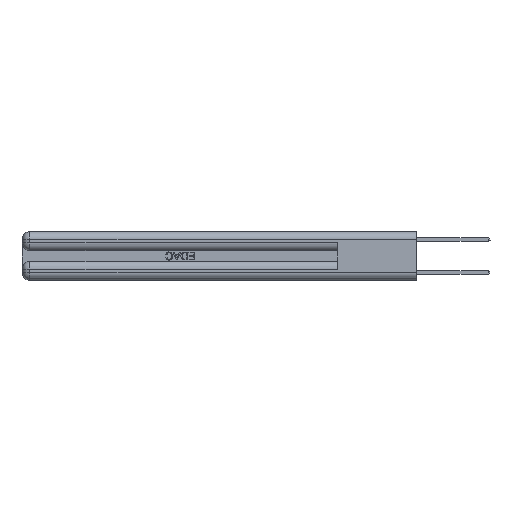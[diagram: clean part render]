
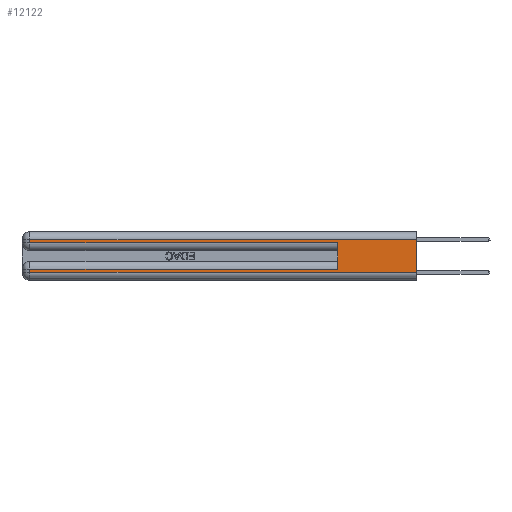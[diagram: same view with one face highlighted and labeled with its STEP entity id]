
A CAD part, left-side view. The second image highlights one B-rep face of the part: STEP entity #12122.
In plain terms, the highlighted planar face has unit normal (-1, 0, 0).
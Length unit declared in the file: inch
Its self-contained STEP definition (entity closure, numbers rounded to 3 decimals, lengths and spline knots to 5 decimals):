
#159 = CARTESIAN_POINT ( 'NONE',  ( 0., 2.94, 0.37 ) ) ;
#1840 = DIRECTION ( 'NONE',  ( 0., -1., 0. ) ) ;
#2116 = DIRECTION ( 'NONE',  ( 0., 1., 0. ) ) ;
#2978 = CARTESIAN_POINT ( 'NONE',  ( 0., 0., 0.285 ) ) ;
#3517 = VECTOR ( 'NONE', #26111, 39.37008 ) ;
#3708 = ORIENTED_EDGE ( 'NONE', *, *, #5303, .T. ) ;
#3730 = EDGE_CURVE ( 'NONE', #18620, #20975, #27559, .T. ) ;
#4450 = ORIENTED_EDGE ( 'NONE', *, *, #28834, .T. ) ;
#4956 = ORIENTED_EDGE ( 'NONE', *, *, #3730, .F. ) ;
#5303 = EDGE_CURVE ( 'NONE', #19756, #13577, #11422, .T. ) ;
#5795 = CARTESIAN_POINT ( 'NONE',  ( 0., 2.94, 0.31 ) ) ;
#6898 = VECTOR ( 'NONE', #15519, 39.37008 ) ;
#7164 = EDGE_CURVE ( 'NONE', #19826, #19756, #14748, .T. ) ;
#7222 = DIRECTION ( 'NONE',  ( 1., 0., 0. ) ) ;
#7768 = CARTESIAN_POINT ( 'NONE',  ( 0., 0.6, 0.285 ) ) ;
#8004 = LINE ( 'NONE', #22572, #20672 ) ;
#11073 = VECTOR ( 'NONE', #16482, 39.37008 ) ;
#11174 = EDGE_CURVE ( 'NONE', #24193, #13577, #8004, .T. ) ;
#11422 = LINE ( 'NONE', #15305, #14850 ) ;
#12122 = ADVANCED_FACE ( 'NONE', ( #18908 ), #23334, .F. ) ;
#12158 = DIRECTION ( 'NONE',  ( 0., 0., -1. ) ) ;
#13145 = ORIENTED_EDGE ( 'NONE', *, *, #7164, .T. ) ;
#13299 = EDGE_CURVE ( 'NONE', #18620, #19826, #31408, .T. ) ;
#13577 = VERTEX_POINT ( 'NONE', #32786 ) ;
#14748 = LINE ( 'NONE', #30093, #24421 ) ;
#14850 = VECTOR ( 'NONE', #1840, 39.37008 ) ;
#15305 = CARTESIAN_POINT ( 'NONE',  ( 0., 0., 0.06 ) ) ;
#15519 = DIRECTION ( 'NONE',  ( 0., 1., 0. ) ) ;
#16013 = VERTEX_POINT ( 'NONE', #28511 ) ;
#16149 = DIRECTION ( 'NONE',  ( 0., 0., 1. ) ) ;
#16348 = VECTOR ( 'NONE', #2116, 39.37008 ) ;
#16482 = DIRECTION ( 'NONE',  ( 0., -1., 0. ) ) ;
#18620 = VERTEX_POINT ( 'NONE', #21579 ) ;
#18908 = FACE_OUTER_BOUND ( 'NONE', #25288, .T. ) ;
#18922 = CARTESIAN_POINT ( 'NONE',  ( 0., 0.6, 0.145 ) ) ;
#19756 = VERTEX_POINT ( 'NONE', #27786 ) ;
#19826 = VERTEX_POINT ( 'NONE', #28006 ) ;
#20258 = DIRECTION ( 'NONE',  ( 0., 0., -1. ) ) ;
#20407 = CARTESIAN_POINT ( 'NONE',  ( 0., 0., 0.085 ) ) ;
#20413 = CARTESIAN_POINT ( 'NONE',  ( 0., 0., 0.37 ) ) ;
#20672 = VECTOR ( 'NONE', #20258, 39.37008 ) ;
#20958 = AXIS2_PLACEMENT_3D ( 'NONE', #20413, #7222, #12158 ) ;
#20975 = VERTEX_POINT ( 'NONE', #7768 ) ;
#21213 = LINE ( 'NONE', #31557, #6898 ) ;
#21248 = VECTOR ( 'NONE', #16149, 39.37008 ) ;
#21579 = CARTESIAN_POINT ( 'NONE',  ( 0., 0.6, 0.085 ) ) ;
#21631 = LINE ( 'NONE', #2978, #11073 ) ;
#21784 = EDGE_CURVE ( 'NONE', #16013, #20975, #21631, .T. ) ;
#22572 = CARTESIAN_POINT ( 'NONE',  ( 0., 0., 0.37 ) ) ;
#23334 = PLANE ( 'NONE',  #20958 ) ;
#24008 = CARTESIAN_POINT ( 'NONE',  ( 0., 0., 0.31 ) ) ;
#24116 = ORIENTED_EDGE ( 'NONE', *, *, #21784, .T. ) ;
#24193 = VERTEX_POINT ( 'NONE', #24008 ) ;
#24421 = VECTOR ( 'NONE', #24862, 39.37008 ) ;
#24862 = DIRECTION ( 'NONE',  ( 0., 0., -1. ) ) ;
#24927 = LINE ( 'NONE', #159, #3517 ) ;
#25288 = EDGE_LOOP ( 'NONE', ( #30430, #29115, #4450, #24116, #4956, #27452, #13145, #3708 ) ) ;
#26111 = DIRECTION ( 'NONE',  ( 0., 0., -1. ) ) ;
#26131 = VERTEX_POINT ( 'NONE', #5795 ) ;
#27452 = ORIENTED_EDGE ( 'NONE', *, *, #13299, .T. ) ;
#27543 = EDGE_CURVE ( 'NONE', #24193, #26131, #21213, .T. ) ;
#27559 = LINE ( 'NONE', #18922, #21248 ) ;
#27786 = CARTESIAN_POINT ( 'NONE',  ( 0., 2.94, 0.06 ) ) ;
#28006 = CARTESIAN_POINT ( 'NONE',  ( 0., 2.94, 0.085 ) ) ;
#28511 = CARTESIAN_POINT ( 'NONE',  ( 0., 2.94, 0.285 ) ) ;
#28834 = EDGE_CURVE ( 'NONE', #26131, #16013, #24927, .T. ) ;
#29115 = ORIENTED_EDGE ( 'NONE', *, *, #27543, .T. ) ;
#30093 = CARTESIAN_POINT ( 'NONE',  ( 0., 2.94, 0.37 ) ) ;
#30430 = ORIENTED_EDGE ( 'NONE', *, *, #11174, .F. ) ;
#31408 = LINE ( 'NONE', #20407, #16348 ) ;
#31557 = CARTESIAN_POINT ( 'NONE',  ( 0., 0., 0.31 ) ) ;
#32786 = CARTESIAN_POINT ( 'NONE',  ( 0., 0., 0.06 ) ) ;
